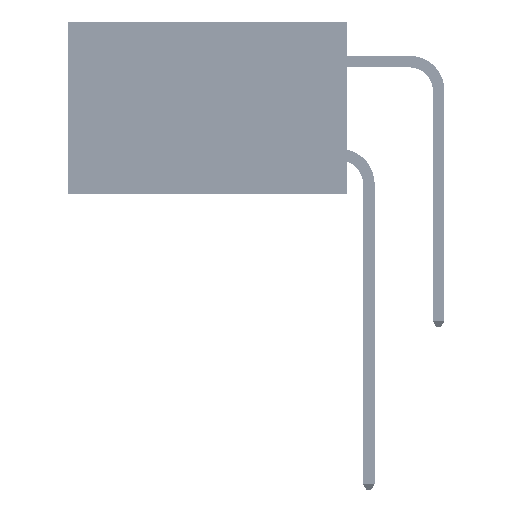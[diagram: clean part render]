
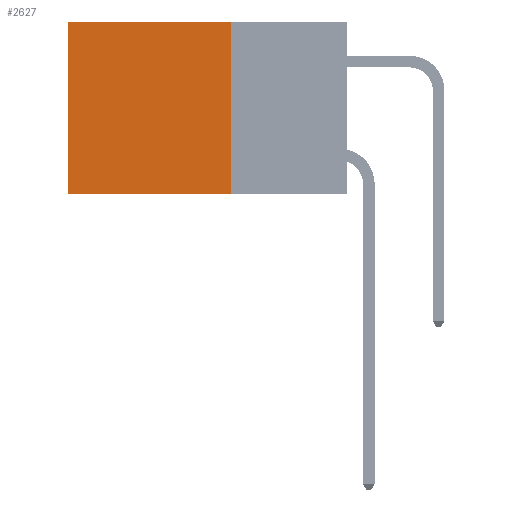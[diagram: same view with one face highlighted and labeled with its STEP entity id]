
A CAD part, left-side view. The second image highlights one B-rep face of the part: STEP entity #2627.
In plain terms, the highlighted planar face has unit normal (-1, 0, 0).
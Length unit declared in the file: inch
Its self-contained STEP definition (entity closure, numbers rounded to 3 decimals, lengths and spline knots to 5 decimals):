
#2627 = ADVANCED_FACE ( 'NONE', ( #20239 ), #43196, .F. ) ;
#3053 = ORIENTED_EDGE ( 'NONE', *, *, #51211, .F. ) ;
#3185 = DIRECTION ( 'NONE',  ( 0., 0., -1. ) ) ;
#3948 = EDGE_CURVE ( 'NONE', #25504, #38888, #44941, .T. ) ;
#6754 = CARTESIAN_POINT ( 'NONE',  ( 0.2875, 0.25, -0.37 ) ) ;
#6940 = LINE ( 'NONE', #27964, #17840 ) ;
#7486 = CARTESIAN_POINT ( 'NONE',  ( 0.2875, 0.25, 0. ) ) ;
#10423 = LINE ( 'NONE', #28589, #51197 ) ;
#12233 = DIRECTION ( 'NONE',  ( 0., 1., 0. ) ) ;
#15237 = LINE ( 'NONE', #17698, #19748 ) ;
#15347 = DIRECTION ( 'NONE',  ( 0., 0., -1. ) ) ;
#15577 = ORIENTED_EDGE ( 'NONE', *, *, #3948, .T. ) ;
#17698 = CARTESIAN_POINT ( 'NONE',  ( 0.2875, 0.25, 0. ) ) ;
#17840 = VECTOR ( 'NONE', #12233, 39.37008 ) ;
#18952 = DIRECTION ( 'NONE',  ( 1., 0., 0. ) ) ;
#19456 = EDGE_LOOP ( 'NONE', ( #15577, #3053, #49608, #41800 ) ) ;
#19748 = VECTOR ( 'NONE', #21636, 39.37008 ) ;
#20069 = DIRECTION ( 'NONE',  ( 0., 0., -1. ) ) ;
#20239 = FACE_OUTER_BOUND ( 'NONE', #19456, .T. ) ;
#21636 = DIRECTION ( 'NONE',  ( 0., 1., 0. ) ) ;
#24562 = VECTOR ( 'NONE', #3185, 39.37008 ) ;
#25024 = AXIS2_PLACEMENT_3D ( 'NONE', #7486, #18952, #15347 ) ;
#25504 = VERTEX_POINT ( 'NONE', #52499 ) ;
#27964 = CARTESIAN_POINT ( 'NONE',  ( 0.2875, 0.25, -0.37 ) ) ;
#28589 = CARTESIAN_POINT ( 'NONE',  ( 0.2875, 0.25, 0. ) ) ;
#29789 = EDGE_CURVE ( 'NONE', #36301, #43253, #10423, .T. ) ;
#33547 = CARTESIAN_POINT ( 'NONE',  ( 0.2875, 0.25, 0. ) ) ;
#36301 = VERTEX_POINT ( 'NONE', #33547 ) ;
#38888 = VERTEX_POINT ( 'NONE', #39721 ) ;
#39721 = CARTESIAN_POINT ( 'NONE',  ( 0.2875, 0.6, -0.37 ) ) ;
#41800 = ORIENTED_EDGE ( 'NONE', *, *, #50983, .T. ) ;
#43196 = PLANE ( 'NONE',  #25024 ) ;
#43253 = VERTEX_POINT ( 'NONE', #6754 ) ;
#44941 = LINE ( 'NONE', #47776, #24562 ) ;
#47776 = CARTESIAN_POINT ( 'NONE',  ( 0.2875, 0.6, 0. ) ) ;
#49608 = ORIENTED_EDGE ( 'NONE', *, *, #29789, .F. ) ;
#50983 = EDGE_CURVE ( 'NONE', #36301, #25504, #15237, .T. ) ;
#51197 = VECTOR ( 'NONE', #20069, 39.37008 ) ;
#51211 = EDGE_CURVE ( 'NONE', #43253, #38888, #6940, .T. ) ;
#52499 = CARTESIAN_POINT ( 'NONE',  ( 0.2875, 0.6, 0. ) ) ;
